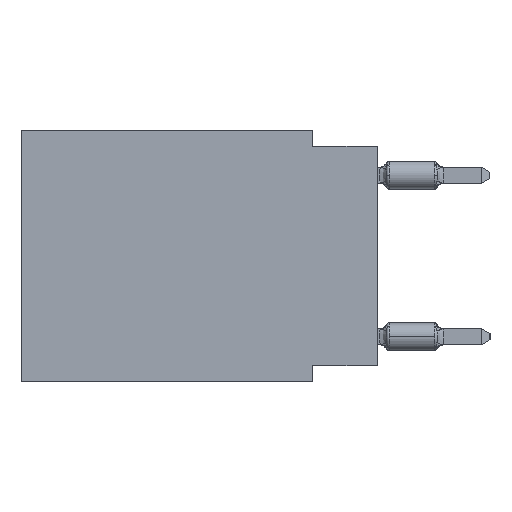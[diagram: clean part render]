
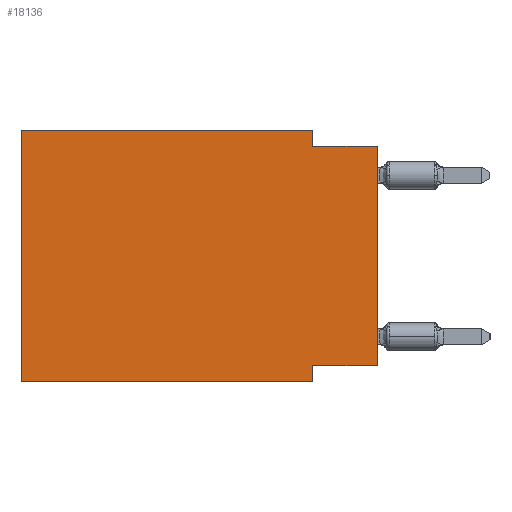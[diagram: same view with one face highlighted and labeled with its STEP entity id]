
A CAD part, left-side view. The second image highlights one B-rep face of the part: STEP entity #18136.
In plain terms, the highlighted planar face has unit normal (-1, 0, 0).
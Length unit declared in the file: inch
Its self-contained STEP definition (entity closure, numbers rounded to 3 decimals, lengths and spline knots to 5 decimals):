
#101 = FACE_OUTER_BOUND ( 'NONE', #22551, .T. ) ;
#1100 = CARTESIAN_POINT ( 'NONE',  ( 0., 0.1, 0. ) ) ;
#1720 = VERTEX_POINT ( 'NONE', #21747 ) ;
#1771 = EDGE_CURVE ( 'NONE', #36240, #23153, #19541, .T. ) ;
#1898 = EDGE_CURVE ( 'NONE', #23153, #28880, #38756, .T. ) ;
#2529 = ORIENTED_EDGE ( 'NONE', *, *, #1898, .F. ) ;
#3899 = DIRECTION ( 'NONE',  ( 0., 0., -1. ) ) ;
#4152 = VECTOR ( 'NONE', #21625, 39.37008 ) ;
#4806 = ORIENTED_EDGE ( 'NONE', *, *, #25732, .F. ) ;
#4964 = CARTESIAN_POINT ( 'NONE',  ( 0., 0.1, -0.025 ) ) ;
#6310 = CARTESIAN_POINT ( 'NONE',  ( 0., 0., -0.365 ) ) ;
#6968 = CARTESIAN_POINT ( 'NONE',  ( 0., 0.1, -0.39 ) ) ;
#7876 = VECTOR ( 'NONE', #18828, 39.37008 ) ;
#9131 = PLANE ( 'NONE',  #36507 ) ;
#9337 = DIRECTION ( 'NONE',  ( 0., 0., -1. ) ) ;
#9993 = DIRECTION ( 'NONE',  ( 0., -1., 0. ) ) ;
#11142 = CARTESIAN_POINT ( 'NONE',  ( 0., 0.55, 0. ) ) ;
#11241 = CARTESIAN_POINT ( 'NONE',  ( 0., 0., -0.025 ) ) ;
#12334 = CARTESIAN_POINT ( 'NONE',  ( 0., 0.55, 0. ) ) ;
#12382 = CARTESIAN_POINT ( 'NONE',  ( 0., 0.55, 0. ) ) ;
#13014 = LINE ( 'NONE', #25211, #7876 ) ;
#13897 = EDGE_CURVE ( 'NONE', #26881, #32073, #31198, .T. ) ;
#14145 = ORIENTED_EDGE ( 'NONE', *, *, #1771, .F. ) ;
#14922 = EDGE_CURVE ( 'NONE', #26354, #28880, #28215, .T. ) ;
#16792 = EDGE_CURVE ( 'NONE', #26354, #27037, #36763, .T. ) ;
#17512 = DIRECTION ( 'NONE',  ( 0., -1., 0. ) ) ;
#17988 = VECTOR ( 'NONE', #17512, 39.37008 ) ;
#18136 = ADVANCED_FACE ( 'NONE', ( #101 ), #9131, .F. ) ;
#18454 = CARTESIAN_POINT ( 'NONE',  ( 0., 0.1, 0. ) ) ;
#18828 = DIRECTION ( 'NONE',  ( 0., 0., -1. ) ) ;
#18964 = EDGE_CURVE ( 'NONE', #26881, #1720, #36396, .T. ) ;
#19184 = CARTESIAN_POINT ( 'NONE',  ( 0., 0.55, -0.39 ) ) ;
#19270 = ORIENTED_EDGE ( 'NONE', *, *, #18964, .F. ) ;
#19541 = LINE ( 'NONE', #1100, #29514 ) ;
#19735 = DIRECTION ( 'NONE',  ( 0., -1., 0. ) ) ;
#20510 = CARTESIAN_POINT ( 'NONE',  ( 0., 0., -0.025 ) ) ;
#21625 = DIRECTION ( 'NONE',  ( 0., 0., 1. ) ) ;
#21747 = CARTESIAN_POINT ( 'NONE',  ( 0., 0.55, 0. ) ) ;
#22551 = EDGE_LOOP ( 'NONE', ( #25631, #2529, #14145, #26971, #19270, #31049, #4806, #23773 ) ) ;
#22939 = LINE ( 'NONE', #11142, #33850 ) ;
#23153 = VERTEX_POINT ( 'NONE', #4964 ) ;
#23773 = ORIENTED_EDGE ( 'NONE', *, *, #16792, .F. ) ;
#24334 = DIRECTION ( 'NONE',  ( 0., 1., 0. ) ) ;
#25211 = CARTESIAN_POINT ( 'NONE',  ( 0., 0.1, -0.39 ) ) ;
#25631 = ORIENTED_EDGE ( 'NONE', *, *, #14922, .T. ) ;
#25732 = EDGE_CURVE ( 'NONE', #27037, #32073, #13014, .T. ) ;
#26354 = VERTEX_POINT ( 'NONE', #32394 ) ;
#26881 = VERTEX_POINT ( 'NONE', #28738 ) ;
#26971 = ORIENTED_EDGE ( 'NONE', *, *, #28025, .F. ) ;
#27037 = VERTEX_POINT ( 'NONE', #37703 ) ;
#27832 = CARTESIAN_POINT ( 'NONE',  ( 0., 0., 0. ) ) ;
#28025 = EDGE_CURVE ( 'NONE', #1720, #36240, #22939, .T. ) ;
#28215 = LINE ( 'NONE', #27832, #4152 ) ;
#28738 = CARTESIAN_POINT ( 'NONE',  ( 0., 0.55, -0.39 ) ) ;
#28880 = VERTEX_POINT ( 'NONE', #11241 ) ;
#29413 = VECTOR ( 'NONE', #24334, 39.37008 ) ;
#29514 = VECTOR ( 'NONE', #3899, 39.37008 ) ;
#31049 = ORIENTED_EDGE ( 'NONE', *, *, #13897, .T. ) ;
#31198 = LINE ( 'NONE', #19184, #38021 ) ;
#32073 = VERTEX_POINT ( 'NONE', #6968 ) ;
#32394 = CARTESIAN_POINT ( 'NONE',  ( 0., 0., -0.365 ) ) ;
#33399 = DIRECTION ( 'NONE',  ( 0., 0., 1. ) ) ;
#33850 = VECTOR ( 'NONE', #19735, 39.37008 ) ;
#34667 = VECTOR ( 'NONE', #33399, 39.37008 ) ;
#36240 = VERTEX_POINT ( 'NONE', #18454 ) ;
#36396 = LINE ( 'NONE', #12382, #34667 ) ;
#36507 = AXIS2_PLACEMENT_3D ( 'NONE', #12334, #36767, #9337 ) ;
#36763 = LINE ( 'NONE', #6310, #29413 ) ;
#36767 = DIRECTION ( 'NONE',  ( 1., 0., 0. ) ) ;
#37703 = CARTESIAN_POINT ( 'NONE',  ( 0., 0.1, -0.365 ) ) ;
#38021 = VECTOR ( 'NONE', #9993, 39.37008 ) ;
#38756 = LINE ( 'NONE', #20510, #17988 ) ;
